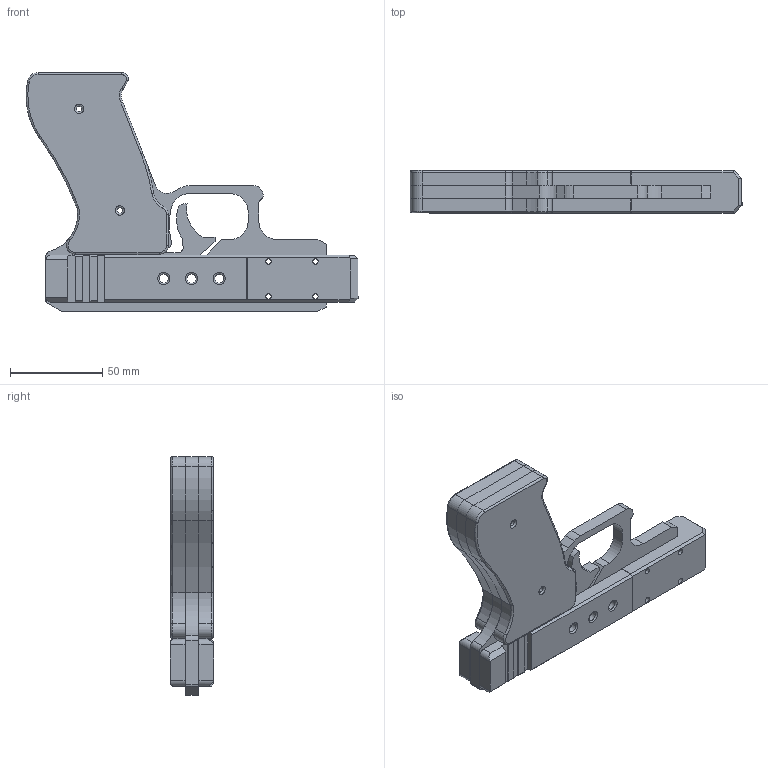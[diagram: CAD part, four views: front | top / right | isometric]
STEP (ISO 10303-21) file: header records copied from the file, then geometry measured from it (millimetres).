
FILE_DESCRIPTION(/* description */ (''),/* implementation_level */ '2;1');
FILE_NAME(/* name */ 'GB 22 ASSEMBLY v7.step',/* time_stamp */ '2021-01-26T03:46:54+01:00',/* author */ (''),/* organization */ (''),/* preprocessor_version */ 'ST-DEVELOPER v18.1',/* originating_system */ 'Autodesk Translation Framework v9.7.1.1290',/* authorisation */ '');
FILE_SCHEMA (('AUTOMOTIVE_DESIGN { 1 0 10303 214 3 1 1 }'));
Length unit declared in the file: millimetre
Products named in the file (8): GB 22 ASSEMBLY; frame GB22; barrel block; bolt middle pice; side bolt block2; side bolt block; grip2; grip
Assembly tree (7 placements, depth 2):
  GB 22 ASSEMBLY
    frame GB22
    barrel block
    bolt middle pice
    side bolt block2
    side bolt block
    grip2
    grip
Bounding box: 179.85 x 23.5 x 129.28 mm (x, y, z)
Volume: 211198.6 mm3; surface area: 78359.9 mm2
Topology: 7 solids, 7 shells, 277 faces, 745 edges, 482 vertices
Faces by surface type: plane 148, cylinder 95, torus 29, cone 5
Full cylindrical faces by diameter (mm): 3 x14, 5 x3, 5.5 x1, 6.2 x5, 6.6 x5
Entity records: 9242 total; most frequent: CARTESIAN_POINT 1753, DIRECTION 1548, ORIENTED_EDGE 1490, EDGE_CURVE 745, AXIS2_PLACEMENT_3D 527, LINE 494, VECTOR 494, VERTEX_POINT 482
